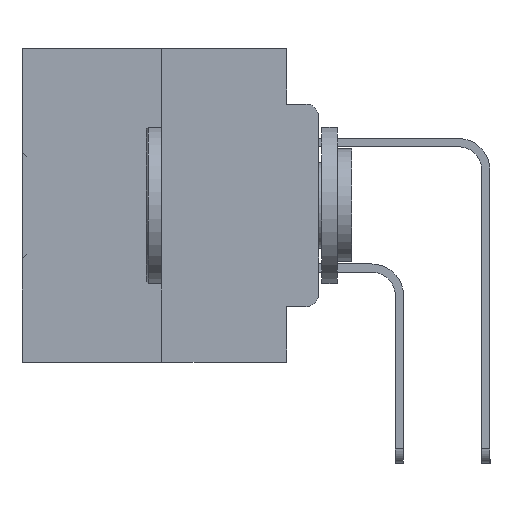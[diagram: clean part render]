
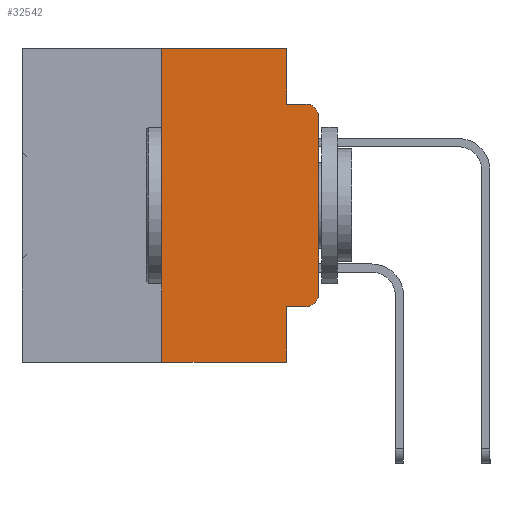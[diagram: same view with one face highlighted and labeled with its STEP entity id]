
A CAD part, left-side view. The second image highlights one B-rep face of the part: STEP entity #32542.
In plain terms, the highlighted planar face has unit normal (-1, 0, 0).
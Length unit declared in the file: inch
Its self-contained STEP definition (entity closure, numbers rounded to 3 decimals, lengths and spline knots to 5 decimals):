
#34 = VECTOR ( 'NONE', #13675, 39.37008 ) ;
#652 = CARTESIAN_POINT ( 'NONE',  ( 0., 0.051, 0. ) ) ;
#665 = DIRECTION ( 'NONE',  ( 0., -1., 0. ) ) ;
#1299 = CARTESIAN_POINT ( 'NONE',  ( 0., 0.051, -0.4115 ) ) ;
#2073 = LINE ( 'NONE', #1299, #31692 ) ;
#2324 = DIRECTION ( 'NONE',  ( -1., 0., 0. ) ) ;
#3301 = LINE ( 'NONE', #15991, #32924 ) ;
#3563 = CIRCLE ( 'NONE', #11191, 0.02 ) ;
#3749 = EDGE_CURVE ( 'NONE', #21713, #29361, #3563, .T. ) ;
#3943 = ORIENTED_EDGE ( 'NONE', *, *, #3749, .T. ) ;
#4294 = CARTESIAN_POINT ( 'NONE',  ( 0., 0., 0. ) ) ;
#6204 = EDGE_CURVE ( 'NONE', #21597, #21743, #35734, .T. ) ;
#7661 = CARTESIAN_POINT ( 'NONE',  ( 0., 0.051, -0.4115 ) ) ;
#7953 = VERTEX_POINT ( 'NONE', #10940 ) ;
#8472 = DIRECTION ( 'NONE',  ( 0., -1., 0. ) ) ;
#9060 = CARTESIAN_POINT ( 'NONE',  ( 0., 0., -0.3915 ) ) ;
#9153 = LINE ( 'NONE', #652, #16785 ) ;
#9622 = EDGE_CURVE ( 'NONE', #13061, #21713, #20777, .T. ) ;
#9711 = PLANE ( 'NONE',  #31266 ) ;
#9864 = ORIENTED_EDGE ( 'NONE', *, *, #16105, .T. ) ;
#9950 = DIRECTION ( 'NONE',  ( 0., -1., 0. ) ) ;
#10884 = ORIENTED_EDGE ( 'NONE', *, *, #37106, .F. ) ;
#10940 = CARTESIAN_POINT ( 'NONE',  ( 0., 0.051, -0.0885 ) ) ;
#11115 = CARTESIAN_POINT ( 'NONE',  ( 0., 0.25, -0.5 ) ) ;
#11191 = AXIS2_PLACEMENT_3D ( 'NONE', #19623, #2324, #22498 ) ;
#11251 = ORIENTED_EDGE ( 'NONE', *, *, #9622, .T. ) ;
#11511 = ORIENTED_EDGE ( 'NONE', *, *, #29530, .F. ) ;
#11687 = VECTOR ( 'NONE', #27886, 39.37008 ) ;
#11979 = ORIENTED_EDGE ( 'NONE', *, *, #6204, .T. ) ;
#13061 = VERTEX_POINT ( 'NONE', #9060 ) ;
#13470 = VECTOR ( 'NONE', #665, 39.37008 ) ;
#13526 = CARTESIAN_POINT ( 'NONE',  ( 0., 0.25, 0. ) ) ;
#13644 = CIRCLE ( 'NONE', #27279, 0.02 ) ;
#13675 = DIRECTION ( 'NONE',  ( 0., -1., 0. ) ) ;
#13939 = CARTESIAN_POINT ( 'NONE',  ( 0., 0.25, 0. ) ) ;
#14797 = VECTOR ( 'NONE', #8472, 39.37008 ) ;
#15477 = DIRECTION ( 'NONE',  ( 0., 0., -1. ) ) ;
#15670 = EDGE_CURVE ( 'NONE', #30950, #20346, #23051, .T. ) ;
#15741 = CARTESIAN_POINT ( 'NONE',  ( 0., 0.02, -0.3915 ) ) ;
#15991 = CARTESIAN_POINT ( 'NONE',  ( 0., 0.051, 0. ) ) ;
#16031 = CARTESIAN_POINT ( 'NONE',  ( 0., 0.051, 0. ) ) ;
#16105 = EDGE_CURVE ( 'NONE', #27813, #13061, #13644, .T. ) ;
#16242 = VERTEX_POINT ( 'NONE', #7661 ) ;
#16785 = VECTOR ( 'NONE', #20836, 39.37008 ) ;
#17734 = FACE_OUTER_BOUND ( 'NONE', #29471, .T. ) ;
#18633 = DIRECTION ( 'NONE',  ( 0., 0., -1. ) ) ;
#19007 = VECTOR ( 'NONE', #27189, 39.37008 ) ;
#19310 = LINE ( 'NONE', #13526, #11687 ) ;
#19429 = CARTESIAN_POINT ( 'NONE',  ( 0., 0.473, 0. ) ) ;
#19623 = CARTESIAN_POINT ( 'NONE',  ( 0., 0.02, -0.1085 ) ) ;
#20070 = ORIENTED_EDGE ( 'NONE', *, *, #23788, .F. ) ;
#20346 = VERTEX_POINT ( 'NONE', #16031 ) ;
#20523 = ORIENTED_EDGE ( 'NONE', *, *, #21886, .T. ) ;
#20777 = LINE ( 'NONE', #4294, #19007 ) ;
#20836 = DIRECTION ( 'NONE',  ( 0., 0., -1. ) ) ;
#20844 = CARTESIAN_POINT ( 'NONE',  ( 0., 0.051, -0.5 ) ) ;
#21597 = VERTEX_POINT ( 'NONE', #11115 ) ;
#21713 = VERTEX_POINT ( 'NONE', #37129 ) ;
#21743 = VERTEX_POINT ( 'NONE', #20844 ) ;
#21886 = EDGE_CURVE ( 'NONE', #16242, #27813, #2073, .T. ) ;
#22498 = DIRECTION ( 'NONE',  ( 0., 0., -1. ) ) ;
#22676 = ORIENTED_EDGE ( 'NONE', *, *, #31415, .F. ) ;
#23051 = LINE ( 'NONE', #19429, #34 ) ;
#23788 = EDGE_CURVE ( 'NONE', #16242, #21743, #9153, .T. ) ;
#24547 = ORIENTED_EDGE ( 'NONE', *, *, #15670, .F. ) ;
#27189 = DIRECTION ( 'NONE',  ( 0., 0., 1. ) ) ;
#27279 = AXIS2_PLACEMENT_3D ( 'NONE', #15741, #35680, #18633 ) ;
#27499 = DIRECTION ( 'NONE',  ( 0., 0., -1. ) ) ;
#27516 = CARTESIAN_POINT ( 'NONE',  ( 0., 0.02, -0.4115 ) ) ;
#27813 = VERTEX_POINT ( 'NONE', #27516 ) ;
#27886 = DIRECTION ( 'NONE',  ( 0., 0., 1. ) ) ;
#29257 = CARTESIAN_POINT ( 'NONE',  ( 0., 0.02, -0.0885 ) ) ;
#29361 = VERTEX_POINT ( 'NONE', #29257 ) ;
#29471 = EDGE_LOOP ( 'NONE', ( #11251, #3943, #10884, #22676, #24547, #11511, #11979, #20070, #20523, #9864 ) ) ;
#29530 = EDGE_CURVE ( 'NONE', #21597, #30950, #19310, .T. ) ;
#29740 = CARTESIAN_POINT ( 'NONE',  ( 0., 0.473, 0. ) ) ;
#30950 = VERTEX_POINT ( 'NONE', #13939 ) ;
#31266 = AXIS2_PLACEMENT_3D ( 'NONE', #29740, #32559, #15477 ) ;
#31415 = EDGE_CURVE ( 'NONE', #20346, #7953, #3301, .T. ) ;
#31692 = VECTOR ( 'NONE', #9950, 39.37008 ) ;
#32542 = ADVANCED_FACE ( 'NONE', ( #17734 ), #9711, .F. ) ;
#32559 = DIRECTION ( 'NONE',  ( 1., 0., 0. ) ) ;
#32924 = VECTOR ( 'NONE', #27499, 39.37008 ) ;
#34214 = CARTESIAN_POINT ( 'NONE',  ( 0., 0.473, -0.5 ) ) ;
#35034 = CARTESIAN_POINT ( 'NONE',  ( 0., 0.051, -0.0885 ) ) ;
#35680 = DIRECTION ( 'NONE',  ( -1., 0., 0. ) ) ;
#35734 = LINE ( 'NONE', #34214, #14797 ) ;
#36206 = LINE ( 'NONE', #35034, #13470 ) ;
#37106 = EDGE_CURVE ( 'NONE', #7953, #29361, #36206, .T. ) ;
#37129 = CARTESIAN_POINT ( 'NONE',  ( 0., 0., -0.1085 ) ) ;
